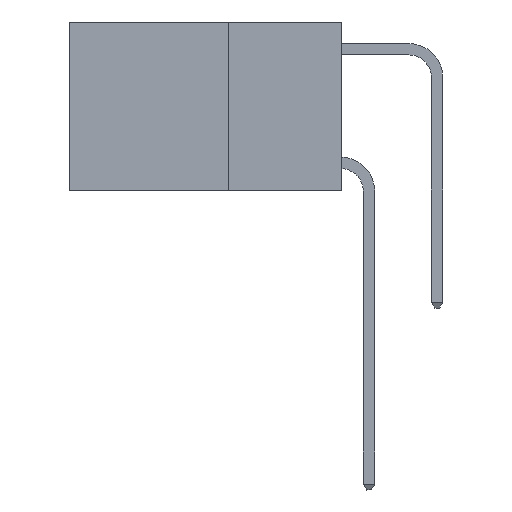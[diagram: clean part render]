
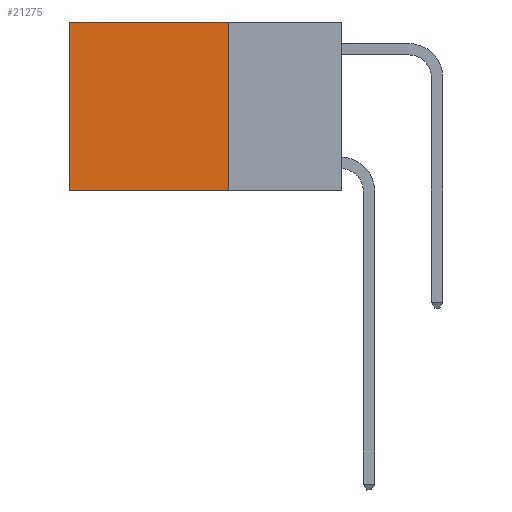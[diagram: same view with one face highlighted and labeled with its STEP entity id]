
A CAD part, left-side view. The second image highlights one B-rep face of the part: STEP entity #21275.
In plain terms, the highlighted planar face has unit normal (-1, 0, 0).
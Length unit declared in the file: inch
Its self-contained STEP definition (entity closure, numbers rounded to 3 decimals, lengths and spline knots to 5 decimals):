
#644 = ORIENTED_EDGE ( 'NONE', *, *, #15547, .T. ) ;
#708 = LINE ( 'NONE', #15999, #13228 ) ;
#771 = EDGE_LOOP ( 'NONE', ( #15258, #17420, #5052, #644 ) ) ;
#1033 = DIRECTION ( 'NONE',  ( 0., 0., -1. ) ) ;
#1382 = EDGE_CURVE ( 'NONE', #14465, #4136, #8947, .T. ) ;
#2403 = CARTESIAN_POINT ( 'NONE',  ( 0.2625, 0.25, -0.37 ) ) ;
#2780 = VECTOR ( 'NONE', #2839, 39.37008 ) ;
#2839 = DIRECTION ( 'NONE',  ( 0., 1., 0. ) ) ;
#3292 = VECTOR ( 'NONE', #3744, 39.37008 ) ;
#3443 = DIRECTION ( 'NONE',  ( 1., 0., 0. ) ) ;
#3744 = DIRECTION ( 'NONE',  ( 0., 1., 0. ) ) ;
#4136 = VERTEX_POINT ( 'NONE', #13199 ) ;
#4883 = DIRECTION ( 'NONE',  ( 0., 0., -1. ) ) ;
#5052 = ORIENTED_EDGE ( 'NONE', *, *, #1382, .F. ) ;
#5101 = PLANE ( 'NONE',  #19568 ) ;
#5348 = EDGE_CURVE ( 'NONE', #5366, #19931, #708, .T. ) ;
#5366 = VERTEX_POINT ( 'NONE', #20865 ) ;
#8544 = CARTESIAN_POINT ( 'NONE',  ( 0.2625, 0.6, -0.37 ) ) ;
#8947 = LINE ( 'NONE', #10687, #11258 ) ;
#10687 = CARTESIAN_POINT ( 'NONE',  ( 0.2625, 0.25, 0. ) ) ;
#11258 = VECTOR ( 'NONE', #15809, 39.37008 ) ;
#12072 = CARTESIAN_POINT ( 'NONE',  ( 0.2625, 0.25, 0. ) ) ;
#13128 = CARTESIAN_POINT ( 'NONE',  ( 0.2625, 0.25, 0. ) ) ;
#13199 = CARTESIAN_POINT ( 'NONE',  ( 0.2625, 0.25, -0.37 ) ) ;
#13228 = VECTOR ( 'NONE', #1033, 39.37008 ) ;
#14465 = VERTEX_POINT ( 'NONE', #21697 ) ;
#15258 = ORIENTED_EDGE ( 'NONE', *, *, #5348, .T. ) ;
#15547 = EDGE_CURVE ( 'NONE', #14465, #5366, #16585, .T. ) ;
#15809 = DIRECTION ( 'NONE',  ( 0., 0., -1. ) ) ;
#15999 = CARTESIAN_POINT ( 'NONE',  ( 0.2625, 0.6, 0. ) ) ;
#16585 = LINE ( 'NONE', #13128, #2780 ) ;
#17420 = ORIENTED_EDGE ( 'NONE', *, *, #19667, .F. ) ;
#19357 = LINE ( 'NONE', #2403, #3292 ) ;
#19568 = AXIS2_PLACEMENT_3D ( 'NONE', #12072, #3443, #4883 ) ;
#19667 = EDGE_CURVE ( 'NONE', #4136, #19931, #19357, .T. ) ;
#19931 = VERTEX_POINT ( 'NONE', #8544 ) ;
#20268 = FACE_OUTER_BOUND ( 'NONE', #771, .T. ) ;
#20865 = CARTESIAN_POINT ( 'NONE',  ( 0.2625, 0.6, 0. ) ) ;
#21275 = ADVANCED_FACE ( 'NONE', ( #20268 ), #5101, .F. ) ;
#21697 = CARTESIAN_POINT ( 'NONE',  ( 0.2625, 0.25, 0. ) ) ;
